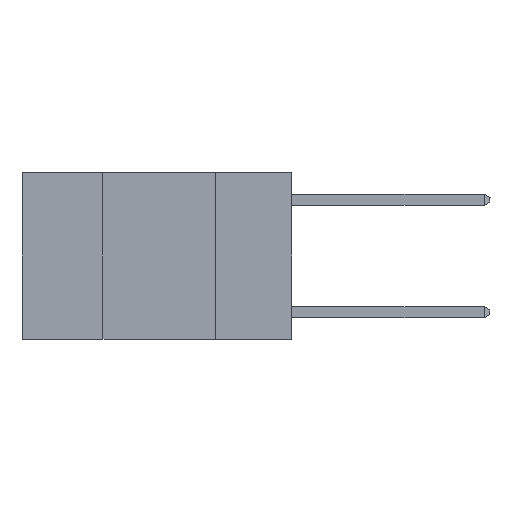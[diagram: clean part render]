
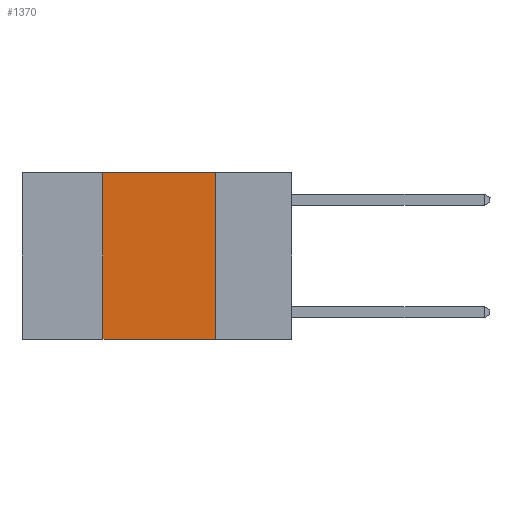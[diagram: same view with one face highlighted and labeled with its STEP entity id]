
A CAD part, left-side view. The second image highlights one B-rep face of the part: STEP entity #1370.
In plain terms, the highlighted planar face has unit normal (-1, 0, 0).
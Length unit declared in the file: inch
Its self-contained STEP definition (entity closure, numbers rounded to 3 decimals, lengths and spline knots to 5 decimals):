
#493 = EDGE_CURVE ( 'NONE', #5083, #13923, #13426, .T. ) ;
#920 = VECTOR ( 'NONE', #13950, 39.37008 ) ;
#1043 = EDGE_CURVE ( 'NONE', #5565, #5083, #4976, .T. ) ;
#1232 = EDGE_CURVE ( 'NONE', #7324, #5565, #16682, .T. ) ;
#1370 = ADVANCED_FACE ( 'NONE', ( #14062 ), #10435, .F. ) ;
#2192 = DIRECTION ( 'NONE',  ( 1., 0., 0. ) ) ;
#2588 = CARTESIAN_POINT ( 'NONE',  ( 0., 0.6, -0.37 ) ) ;
#2917 = CARTESIAN_POINT ( 'NONE',  ( 0., 0.6, 0. ) ) ;
#3859 = AXIS2_PLACEMENT_3D ( 'NONE', #15916, #2192, #11785 ) ;
#4861 = EDGE_LOOP ( 'NONE', ( #10024, #11011, #12421, #12579 ) ) ;
#4976 = LINE ( 'NONE', #2917, #920 ) ;
#4994 = VECTOR ( 'NONE', #9452, 39.37008 ) ;
#5083 = VERTEX_POINT ( 'NONE', #7000 ) ;
#5565 = VERTEX_POINT ( 'NONE', #8091 ) ;
#5630 = VECTOR ( 'NONE', #14296, 39.37008 ) ;
#7000 = CARTESIAN_POINT ( 'NONE',  ( 0., 0.17, 0. ) ) ;
#7273 = DIRECTION ( 'NONE',  ( 0., 0., -1. ) ) ;
#7324 = VERTEX_POINT ( 'NONE', #13537 ) ;
#8091 = CARTESIAN_POINT ( 'NONE',  ( 0., 0.42, 0. ) ) ;
#9452 = DIRECTION ( 'NONE',  ( 0., -1., 0. ) ) ;
#10000 = LINE ( 'NONE', #2588, #4994 ) ;
#10024 = ORIENTED_EDGE ( 'NONE', *, *, #493, .F. ) ;
#10134 = CARTESIAN_POINT ( 'NONE',  ( 0., 0.42, 0. ) ) ;
#10184 = VECTOR ( 'NONE', #7273, 39.37008 ) ;
#10435 = PLANE ( 'NONE',  #3859 ) ;
#11011 = ORIENTED_EDGE ( 'NONE', *, *, #1043, .F. ) ;
#11785 = DIRECTION ( 'NONE',  ( 0., 0., -1. ) ) ;
#12421 = ORIENTED_EDGE ( 'NONE', *, *, #1232, .F. ) ;
#12579 = ORIENTED_EDGE ( 'NONE', *, *, #13128, .T. ) ;
#13128 = EDGE_CURVE ( 'NONE', #7324, #13923, #10000, .T. ) ;
#13426 = LINE ( 'NONE', #16935, #10184 ) ;
#13537 = CARTESIAN_POINT ( 'NONE',  ( 0., 0.42, -0.37 ) ) ;
#13923 = VERTEX_POINT ( 'NONE', #16558 ) ;
#13950 = DIRECTION ( 'NONE',  ( 0., -1., 0. ) ) ;
#14062 = FACE_OUTER_BOUND ( 'NONE', #4861, .T. ) ;
#14296 = DIRECTION ( 'NONE',  ( 0., 0., 1. ) ) ;
#15916 = CARTESIAN_POINT ( 'NONE',  ( 0., 0.6, 0. ) ) ;
#16558 = CARTESIAN_POINT ( 'NONE',  ( 0., 0.17, -0.37 ) ) ;
#16682 = LINE ( 'NONE', #10134, #5630 ) ;
#16935 = CARTESIAN_POINT ( 'NONE',  ( 0., 0.17, 0. ) ) ;
